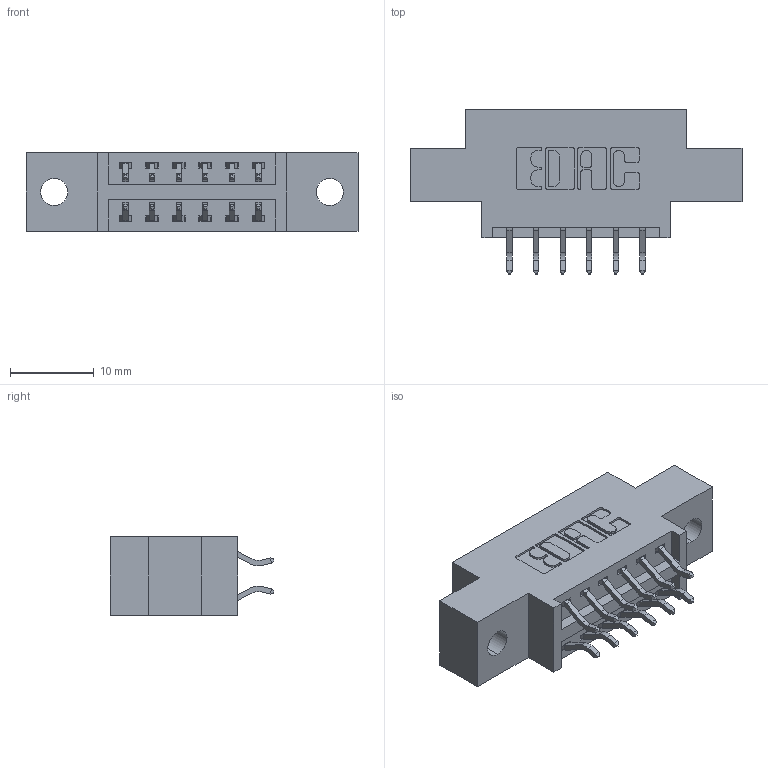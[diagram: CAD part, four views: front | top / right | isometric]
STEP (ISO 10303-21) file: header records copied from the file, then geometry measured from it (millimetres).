
FILE_DESCRIPTION (( 'STEP AP203' ), '1' );
FILE_NAME ('396-012-556-802.STEP', '2019-11-01T17:06:27', ( '' ), ( '' ), 'SwSTEP 2.0', 'SolidWorks 2016', '' );
FILE_SCHEMA (( 'CONFIG_CONTROL_DESIGN' ));
Length unit declared in the file: inch
Products named in the file (3): 345-292-001_556 Tail; 396-012-556-802; 346 Part_0.170 Offset - 0.128 Dia
Assembly tree (13 placements, depth 2):
  396-012-556-802
    346 Part_0.170 Offset - 0.128 Dia
    345-292-001_556 Tail  x12
Bounding box: 39.62 x 19.57 x 9.4 mm (x, y, z)
Volume: 3392.5 mm3; surface area: 3996.5 mm2
Topology: 13 solids, 13 shells, 822 faces, 2417 edges, 1594 vertices
Faces by surface type: plane 548, cylinder 274
Entity records: 9117 total; most frequent: CARTESIAN_POINT 1568, ORIENTED_EDGE 1490, DIRECTION 1421, EDGE_CURVE 745, LINE 581, VECTOR 581, VERTEX_POINT 494, AXIS2_PLACEMENT_3D 420
